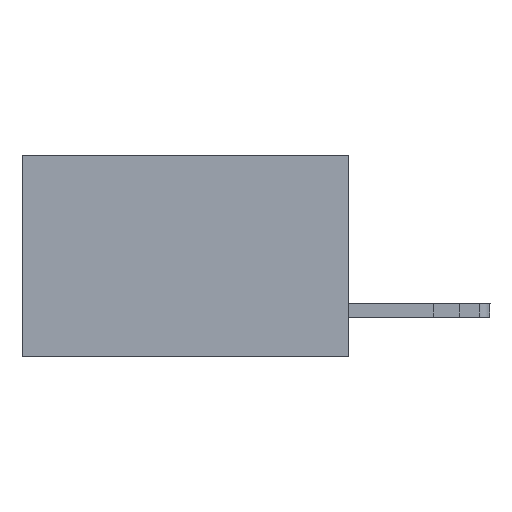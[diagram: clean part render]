
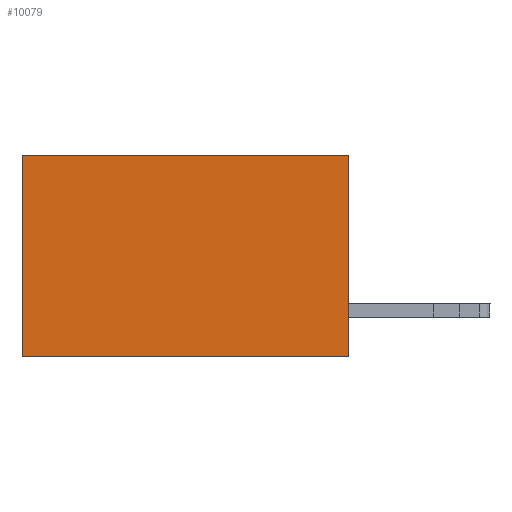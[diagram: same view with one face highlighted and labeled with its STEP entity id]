
A CAD part, left-side view. The second image highlights one B-rep face of the part: STEP entity #10079.
In plain terms, the highlighted planar face has unit normal (-1, 0, 0).
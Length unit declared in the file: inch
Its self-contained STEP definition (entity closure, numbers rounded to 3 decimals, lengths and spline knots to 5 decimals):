
#41 = EDGE_CURVE ( 'NONE', #9134, #8540, #11763, .T. ) ;
#94 = CARTESIAN_POINT ( 'NONE',  ( 0.298, 0.6, 0. ) ) ;
#272 = CARTESIAN_POINT ( 'NONE',  ( 0.298, 0.6, -0.37 ) ) ;
#283 = DIRECTION ( 'NONE',  ( 0., 0., -1. ) ) ;
#488 = ORIENTED_EDGE ( 'NONE', *, *, #41, .F. ) ;
#535 = DIRECTION ( 'NONE',  ( 0., 1., 0. ) ) ;
#971 = CARTESIAN_POINT ( 'NONE',  ( 0.298, 0., -0.37 ) ) ;
#1541 = LINE ( 'NONE', #5587, #6992 ) ;
#1582 = CARTESIAN_POINT ( 'NONE',  ( 0.298, 0., 0. ) ) ;
#2033 = LINE ( 'NONE', #971, #12062 ) ;
#3757 = DIRECTION ( 'NONE',  ( 0., 0., -1. ) ) ;
#4096 = VECTOR ( 'NONE', #4199, 39.37008 ) ;
#4199 = DIRECTION ( 'NONE',  ( 0., 0., -1. ) ) ;
#4286 = AXIS2_PLACEMENT_3D ( 'NONE', #11538, #4593, #283 ) ;
#4519 = VERTEX_POINT ( 'NONE', #272 ) ;
#4593 = DIRECTION ( 'NONE',  ( 1., 0., 0. ) ) ;
#5093 = EDGE_LOOP ( 'NONE', ( #6438, #11454, #488, #10737 ) ) ;
#5202 = LINE ( 'NONE', #94, #4096 ) ;
#5279 = CARTESIAN_POINT ( 'NONE',  ( 0.298, 0.6, 0. ) ) ;
#5479 = CARTESIAN_POINT ( 'NONE',  ( 0.298, 0., -0.37 ) ) ;
#5587 = CARTESIAN_POINT ( 'NONE',  ( 0.298, 0., 0. ) ) ;
#6438 = ORIENTED_EDGE ( 'NONE', *, *, #12709, .T. ) ;
#6992 = VECTOR ( 'NONE', #535, 39.37008 ) ;
#7441 = FACE_OUTER_BOUND ( 'NONE', #5093, .T. ) ;
#7572 = PLANE ( 'NONE',  #4286 ) ;
#8158 = CARTESIAN_POINT ( 'NONE',  ( 0.298, 0., 0. ) ) ;
#8540 = VERTEX_POINT ( 'NONE', #5479 ) ;
#9022 = EDGE_CURVE ( 'NONE', #9134, #10907, #1541, .T. ) ;
#9134 = VERTEX_POINT ( 'NONE', #8158 ) ;
#9313 = DIRECTION ( 'NONE',  ( 0., 1., 0. ) ) ;
#9665 = EDGE_CURVE ( 'NONE', #8540, #4519, #2033, .T. ) ;
#9972 = VECTOR ( 'NONE', #3757, 39.37008 ) ;
#10079 = ADVANCED_FACE ( 'NONE', ( #7441 ), #7572, .F. ) ;
#10737 = ORIENTED_EDGE ( 'NONE', *, *, #9022, .T. ) ;
#10907 = VERTEX_POINT ( 'NONE', #5279 ) ;
#11454 = ORIENTED_EDGE ( 'NONE', *, *, #9665, .F. ) ;
#11538 = CARTESIAN_POINT ( 'NONE',  ( 0.298, 0., 0. ) ) ;
#11763 = LINE ( 'NONE', #1582, #9972 ) ;
#12062 = VECTOR ( 'NONE', #9313, 39.37008 ) ;
#12709 = EDGE_CURVE ( 'NONE', #10907, #4519, #5202, .T. ) ;
